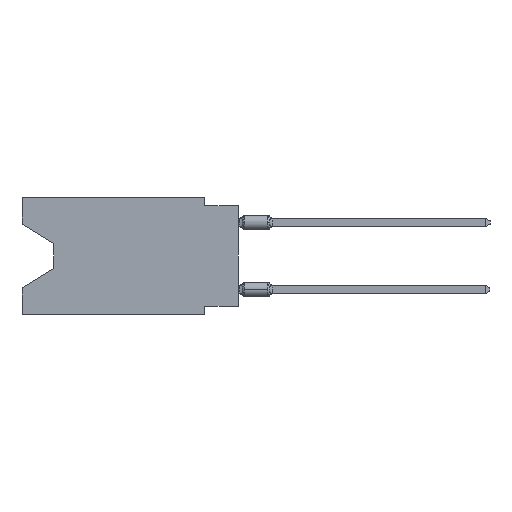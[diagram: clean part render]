
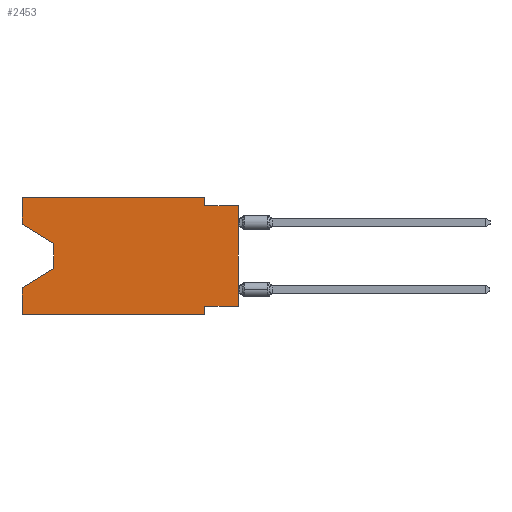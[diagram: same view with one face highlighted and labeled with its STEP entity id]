
A CAD part, left-side view. The second image highlights one B-rep face of the part: STEP entity #2453.
In plain terms, the highlighted planar face has unit normal (-1, 0, 0).
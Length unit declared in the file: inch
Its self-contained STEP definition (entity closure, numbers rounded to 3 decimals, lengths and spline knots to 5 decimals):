
#608 = VERTEX_POINT ( 'NONE', #43516 ) ;
#1441 = CARTESIAN_POINT ( 'NONE',  ( 0., 0.1, -0.35 ) ) ;
#1557 = VERTEX_POINT ( 'NONE', #24732 ) ;
#2453 = ADVANCED_FACE ( 'NONE', ( #40066 ), #19109, .F. ) ;
#3266 = LINE ( 'NONE', #24204, #20281 ) ;
#3660 = EDGE_CURVE ( 'NONE', #13438, #7053, #7797, .T. ) ;
#3951 = DIRECTION ( 'NONE',  ( 0., 0., 1. ) ) ;
#4586 = CARTESIAN_POINT ( 'NONE',  ( 0., 0., -0.025 ) ) ;
#4995 = CARTESIAN_POINT ( 'NONE',  ( 0., 0.1, -0.025 ) ) ;
#5747 = DIRECTION ( 'NONE',  ( 0., 0., -1. ) ) ;
#5871 = ORIENTED_EDGE ( 'NONE', *, *, #40002, .T. ) ;
#6330 = ORIENTED_EDGE ( 'NONE', *, *, #23054, .F. ) ;
#6970 = CARTESIAN_POINT ( 'NONE',  ( 0., 0., -0.025 ) ) ;
#7053 = VERTEX_POINT ( 'NONE', #4995 ) ;
#7180 = CARTESIAN_POINT ( 'NONE',  ( 0., 0., 0. ) ) ;
#7797 = LINE ( 'NONE', #32515, #45363 ) ;
#7891 = VERTEX_POINT ( 'NONE', #20069 ) ;
#8418 = AXIS2_PLACEMENT_3D ( 'NONE', #31190, #31719, #45083 ) ;
#8570 = CARTESIAN_POINT ( 'NONE',  ( 0., 0.55, -0.138 ) ) ;
#8625 = LINE ( 'NONE', #4586, #37228 ) ;
#9684 = DIRECTION ( 'NONE',  ( 0., -1., 0. ) ) ;
#9754 = LINE ( 'NONE', #39050, #36421 ) ;
#10169 = VECTOR ( 'NONE', #29494, 39.37008 ) ;
#10227 = LINE ( 'NONE', #30109, #36358 ) ;
#11238 = LINE ( 'NONE', #7180, #13725 ) ;
#11889 = DIRECTION ( 'NONE',  ( 0., 0., 1. ) ) ;
#11893 = VERTEX_POINT ( 'NONE', #12072 ) ;
#11952 = DIRECTION ( 'NONE',  ( 0., 0.855, -0.519 ) ) ;
#12072 = CARTESIAN_POINT ( 'NONE',  ( 0., 0.645, -0.26975 ) ) ;
#12555 = CARTESIAN_POINT ( 'NONE',  ( 0., 0.645, -0.08025 ) ) ;
#13438 = VERTEX_POINT ( 'NONE', #31108 ) ;
#13519 = EDGE_CURVE ( 'NONE', #7053, #18630, #8625, .T. ) ;
#13725 = VECTOR ( 'NONE', #3951, 39.37008 ) ;
#14437 = EDGE_CURVE ( 'NONE', #38065, #11893, #26745, .T. ) ;
#14591 = ORIENTED_EDGE ( 'NONE', *, *, #13519, .F. ) ;
#15813 = EDGE_CURVE ( 'NONE', #1557, #17843, #3266, .T. ) ;
#16300 = LINE ( 'NONE', #12555, #44886 ) ;
#17655 = VERTEX_POINT ( 'NONE', #8570 ) ;
#17843 = VERTEX_POINT ( 'NONE', #31620 ) ;
#17968 = VERTEX_POINT ( 'NONE', #23037 ) ;
#18630 = VERTEX_POINT ( 'NONE', #6970 ) ;
#19109 = PLANE ( 'NONE',  #8418 ) ;
#19206 = EDGE_CURVE ( 'NONE', #1557, #17655, #16300, .T. ) ;
#19675 = EDGE_CURVE ( 'NONE', #17843, #13438, #10227, .T. ) ;
#20069 = CARTESIAN_POINT ( 'NONE',  ( 0., 0., -0.325 ) ) ;
#20271 = ORIENTED_EDGE ( 'NONE', *, *, #49600, .F. ) ;
#20281 = VECTOR ( 'NONE', #41140, 39.37008 ) ;
#20303 = ORIENTED_EDGE ( 'NONE', *, *, #19206, .T. ) ;
#20459 = DIRECTION ( 'NONE',  ( 0., -1., 0. ) ) ;
#20466 = DIRECTION ( 'NONE',  ( 0., 0., -1. ) ) ;
#21870 = LINE ( 'NONE', #1441, #47008 ) ;
#23037 = CARTESIAN_POINT ( 'NONE',  ( 0., 0.645, -0.35 ) ) ;
#23054 = EDGE_CURVE ( 'NONE', #17968, #11893, #23959, .T. ) ;
#23959 = LINE ( 'NONE', #36574, #51187 ) ;
#24204 = CARTESIAN_POINT ( 'NONE',  ( 0., 0.645, 0. ) ) ;
#24464 = DIRECTION ( 'NONE',  ( 0., 0., -1. ) ) ;
#24732 = CARTESIAN_POINT ( 'NONE',  ( 0., 0.645, -0.08025 ) ) ;
#25908 = EDGE_CURVE ( 'NONE', #7891, #18630, #11238, .T. ) ;
#26745 = LINE ( 'NONE', #43144, #39068 ) ;
#29058 = CARTESIAN_POINT ( 'NONE',  ( 0., 0.55, -0.138 ) ) ;
#29494 = DIRECTION ( 'NONE',  ( 0., 1., 0. ) ) ;
#30031 = LINE ( 'NONE', #46397, #10169 ) ;
#30109 = CARTESIAN_POINT ( 'NONE',  ( 0., 0.645, 0. ) ) ;
#31108 = CARTESIAN_POINT ( 'NONE',  ( 0., 0.1, 0. ) ) ;
#31190 = CARTESIAN_POINT ( 'NONE',  ( 0., 0.645, 0. ) ) ;
#31620 = CARTESIAN_POINT ( 'NONE',  ( 0., 0.645, 0. ) ) ;
#31719 = DIRECTION ( 'NONE',  ( 1., 0., 0. ) ) ;
#32515 = CARTESIAN_POINT ( 'NONE',  ( 0., 0.1, 0. ) ) ;
#33530 = ORIENTED_EDGE ( 'NONE', *, *, #43312, .F. ) ;
#35905 = ORIENTED_EDGE ( 'NONE', *, *, #3660, .F. ) ;
#36358 = VECTOR ( 'NONE', #9684, 39.37008 ) ;
#36421 = VECTOR ( 'NONE', #50863, 39.37008 ) ;
#36574 = CARTESIAN_POINT ( 'NONE',  ( 0., 0.645, 0. ) ) ;
#37228 = VECTOR ( 'NONE', #20459, 39.37008 ) ;
#37376 = LINE ( 'NONE', #29058, #48430 ) ;
#37557 = EDGE_CURVE ( 'NONE', #17655, #38065, #37376, .T. ) ;
#37891 = VERTEX_POINT ( 'NONE', #49690 ) ;
#38065 = VERTEX_POINT ( 'NONE', #42416 ) ;
#39050 = CARTESIAN_POINT ( 'NONE',  ( 0., 0.645, -0.35 ) ) ;
#39068 = VECTOR ( 'NONE', #11952, 39.37008 ) ;
#40002 = EDGE_CURVE ( 'NONE', #17968, #608, #9754, .T. ) ;
#40066 = FACE_OUTER_BOUND ( 'NONE', #46965, .T. ) ;
#41140 = DIRECTION ( 'NONE',  ( 0., 0., 1. ) ) ;
#42416 = CARTESIAN_POINT ( 'NONE',  ( 0., 0.55, -0.212 ) ) ;
#43144 = CARTESIAN_POINT ( 'NONE',  ( 0., 0.55, -0.212 ) ) ;
#43167 = ORIENTED_EDGE ( 'NONE', *, *, #37557, .T. ) ;
#43312 = EDGE_CURVE ( 'NONE', #37891, #608, #21870, .T. ) ;
#43333 = ORIENTED_EDGE ( 'NONE', *, *, #15813, .F. ) ;
#43516 = CARTESIAN_POINT ( 'NONE',  ( 0., 0.1, -0.35 ) ) ;
#44270 = ORIENTED_EDGE ( 'NONE', *, *, #19675, .F. ) ;
#44886 = VECTOR ( 'NONE', #48558, 39.37008 ) ;
#45083 = DIRECTION ( 'NONE',  ( 0., 0., -1. ) ) ;
#45363 = VECTOR ( 'NONE', #24464, 39.37008 ) ;
#46397 = CARTESIAN_POINT ( 'NONE',  ( 0., 0., -0.325 ) ) ;
#46965 = EDGE_LOOP ( 'NONE', ( #20303, #43167, #49910, #6330, #5871, #33530, #20271, #51384, #14591, #35905, #44270, #43333 ) ) ;
#47008 = VECTOR ( 'NONE', #5747, 39.37008 ) ;
#48430 = VECTOR ( 'NONE', #20466, 39.37008 ) ;
#48558 = DIRECTION ( 'NONE',  ( 0., -0.855, -0.519 ) ) ;
#49600 = EDGE_CURVE ( 'NONE', #7891, #37891, #30031, .T. ) ;
#49690 = CARTESIAN_POINT ( 'NONE',  ( 0., 0.1, -0.325 ) ) ;
#49910 = ORIENTED_EDGE ( 'NONE', *, *, #14437, .T. ) ;
#50863 = DIRECTION ( 'NONE',  ( 0., -1., 0. ) ) ;
#51187 = VECTOR ( 'NONE', #11889, 39.37008 ) ;
#51384 = ORIENTED_EDGE ( 'NONE', *, *, #25908, .T. ) ;
